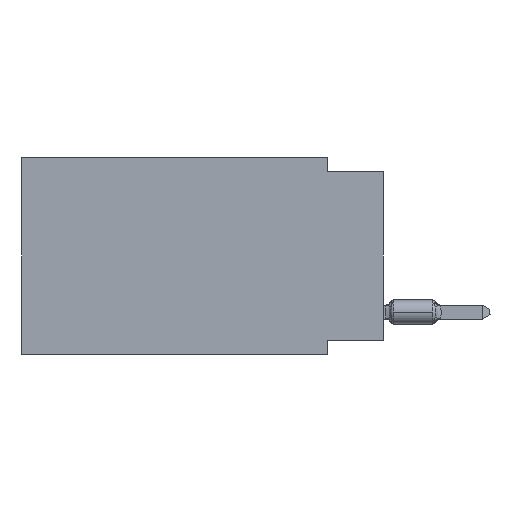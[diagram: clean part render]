
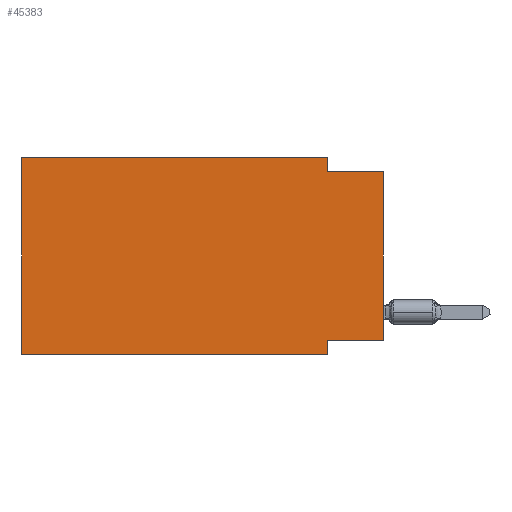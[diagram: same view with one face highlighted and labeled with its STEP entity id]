
A CAD part, left-side view. The second image highlights one B-rep face of the part: STEP entity #45383.
In plain terms, the highlighted planar face has unit normal (-1, 0, 0).
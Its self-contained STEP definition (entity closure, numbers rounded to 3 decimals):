
#767 = CARTESIAN_POINT ( 'NONE',  ( 0., 0., 0. ) ) ;
#1174 = VERTEX_POINT ( 'NONE', #15215 ) ;
#1727 = VECTOR ( 'NONE', #56144, 1000. ) ;
#2590 = ORIENTED_EDGE ( 'NONE', *, *, #14683, .F. ) ;
#3133 = EDGE_CURVE ( 'NONE', #4565, #1174, #58901, .T. ) ;
#4565 = VERTEX_POINT ( 'NONE', #44610 ) ;
#4913 = EDGE_LOOP ( 'NONE', ( #28571, #11354, #9577, #49249, #34313, #57821, #2590, #34165 ) ) ;
#7015 = CARTESIAN_POINT ( 'NONE',  ( 0., 16.383, -8.89 ) ) ;
#7445 = LINE ( 'NONE', #54622, #55602 ) ;
#8106 = VECTOR ( 'NONE', #55359, 1000. ) ;
#8859 = CARTESIAN_POINT ( 'NONE',  ( 0., 2.54, -8.89 ) ) ;
#9577 = ORIENTED_EDGE ( 'NONE', *, *, #53214, .F. ) ;
#10663 = DIRECTION ( 'NONE',  ( 0., -1., 0. ) ) ;
#11354 = ORIENTED_EDGE ( 'NONE', *, *, #42041, .F. ) ;
#12011 = CARTESIAN_POINT ( 'NONE',  ( 0., 0., -0.635 ) ) ;
#12311 = VERTEX_POINT ( 'NONE', #12011 ) ;
#13567 = VECTOR ( 'NONE', #57338, 1000. ) ;
#13646 = CARTESIAN_POINT ( 'NONE',  ( 0., 2.54, 0. ) ) ;
#14683 = EDGE_CURVE ( 'NONE', #1174, #49584, #33763, .T. ) ;
#15215 = CARTESIAN_POINT ( 'NONE',  ( 0., 2.54, -8.255 ) ) ;
#16415 = EDGE_CURVE ( 'NONE', #40001, #49584, #50043, .T. ) ;
#17143 = VERTEX_POINT ( 'NONE', #57738 ) ;
#17414 = VERTEX_POINT ( 'NONE', #17928 ) ;
#17733 = DIRECTION ( 'NONE',  ( 0., -1., 0. ) ) ;
#17928 = CARTESIAN_POINT ( 'NONE',  ( 0., 16.383, 0. ) ) ;
#18299 = CARTESIAN_POINT ( 'NONE',  ( 0., 2.54, 0. ) ) ;
#21066 = CARTESIAN_POINT ( 'NONE',  ( 0., 0., -8.255 ) ) ;
#21195 = DIRECTION ( 'NONE',  ( 0., 0., -1. ) ) ;
#22266 = VECTOR ( 'NONE', #10663, 1000. ) ;
#22979 = LINE ( 'NONE', #18299, #23311 ) ;
#23311 = VECTOR ( 'NONE', #56123, 1000. ) ;
#27754 = VECTOR ( 'NONE', #21195, 1000. ) ;
#28425 = VECTOR ( 'NONE', #57681, 1000. ) ;
#28571 = ORIENTED_EDGE ( 'NONE', *, *, #56140, .T. ) ;
#29317 = VERTEX_POINT ( 'NONE', #13646 ) ;
#30522 = PLANE ( 'NONE',  #55578 ) ;
#31127 = CARTESIAN_POINT ( 'NONE',  ( 0., 16.383, 0. ) ) ;
#33489 = CARTESIAN_POINT ( 'NONE',  ( 0., 0., -0.635 ) ) ;
#33763 = LINE ( 'NONE', #52523, #27754 ) ;
#34165 = ORIENTED_EDGE ( 'NONE', *, *, #3133, .F. ) ;
#34313 = ORIENTED_EDGE ( 'NONE', *, *, #35503, .F. ) ;
#35503 = EDGE_CURVE ( 'NONE', #40001, #17414, #52071, .T. ) ;
#36569 = EDGE_CURVE ( 'NONE', #17414, #29317, #7445, .T. ) ;
#40001 = VERTEX_POINT ( 'NONE', #7015 ) ;
#40825 = DIRECTION ( 'NONE',  ( 1., 0., 0. ) ) ;
#42041 = EDGE_CURVE ( 'NONE', #17143, #12311, #48464, .T. ) ;
#44610 = CARTESIAN_POINT ( 'NONE',  ( 0., 0., -8.255 ) ) ;
#44885 = FACE_OUTER_BOUND ( 'NONE', #4913, .T. ) ;
#45383 = ADVANCED_FACE ( 'NONE', ( #44885 ), #30522, .F. ) ;
#48464 = LINE ( 'NONE', #33489, #22266 ) ;
#49249 = ORIENTED_EDGE ( 'NONE', *, *, #36569, .F. ) ;
#49584 = VERTEX_POINT ( 'NONE', #8859 ) ;
#50043 = LINE ( 'NONE', #59106, #8106 ) ;
#52071 = LINE ( 'NONE', #56779, #1727 ) ;
#52523 = CARTESIAN_POINT ( 'NONE',  ( 0., 2.54, -8.89 ) ) ;
#53214 = EDGE_CURVE ( 'NONE', #29317, #17143, #22979, .T. ) ;
#54622 = CARTESIAN_POINT ( 'NONE',  ( 0., 16.383, 0. ) ) ;
#55359 = DIRECTION ( 'NONE',  ( 0., -1., 0. ) ) ;
#55578 = AXIS2_PLACEMENT_3D ( 'NONE', #31127, #40825, #59872 ) ;
#55602 = VECTOR ( 'NONE', #17733, 1000. ) ;
#56123 = DIRECTION ( 'NONE',  ( 0., 0., -1. ) ) ;
#56140 = EDGE_CURVE ( 'NONE', #4565, #12311, #56739, .T. ) ;
#56144 = DIRECTION ( 'NONE',  ( 0., 0., 1. ) ) ;
#56739 = LINE ( 'NONE', #767, #13567 ) ;
#56779 = CARTESIAN_POINT ( 'NONE',  ( 0., 16.383, 0. ) ) ;
#57338 = DIRECTION ( 'NONE',  ( 0., 0., 1. ) ) ;
#57681 = DIRECTION ( 'NONE',  ( 0., 1., 0. ) ) ;
#57738 = CARTESIAN_POINT ( 'NONE',  ( 0., 2.54, -0.635 ) ) ;
#57821 = ORIENTED_EDGE ( 'NONE', *, *, #16415, .T. ) ;
#58901 = LINE ( 'NONE', #21066, #28425 ) ;
#59106 = CARTESIAN_POINT ( 'NONE',  ( 0., 16.383, -8.89 ) ) ;
#59872 = DIRECTION ( 'NONE',  ( 0., 0., -1. ) ) ;
